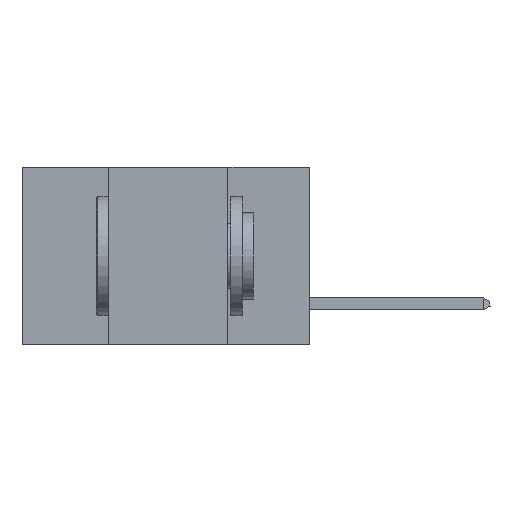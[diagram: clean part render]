
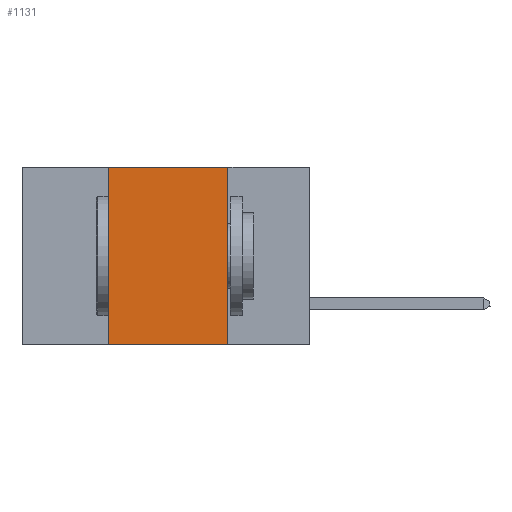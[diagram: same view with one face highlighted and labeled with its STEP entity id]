
A CAD part, left-side view. The second image highlights one B-rep face of the part: STEP entity #1131.
In plain terms, the highlighted planar face has unit normal (-1, 0, 0).
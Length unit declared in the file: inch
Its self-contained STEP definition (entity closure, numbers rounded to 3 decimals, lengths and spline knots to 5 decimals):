
#219 = VERTEX_POINT ( 'NONE', #9685 ) ;
#1131 = ADVANCED_FACE ( 'NONE', ( #25147 ), #12726, .F. ) ;
#2560 = CARTESIAN_POINT ( 'NONE',  ( 0., 0.42, 0. ) ) ;
#2862 = DIRECTION ( 'NONE',  ( 0., -1., 0. ) ) ;
#3616 = ORIENTED_EDGE ( 'NONE', *, *, #7091, .T. ) ;
#6191 = LINE ( 'NONE', #12866, #13840 ) ;
#6233 = DIRECTION ( 'NONE',  ( 0., 0., -1. ) ) ;
#6569 = DIRECTION ( 'NONE',  ( 0., 0., 1. ) ) ;
#7091 = EDGE_CURVE ( 'NONE', #219, #16683, #10833, .T. ) ;
#7781 = VERTEX_POINT ( 'NONE', #19347 ) ;
#8742 = CARTESIAN_POINT ( 'NONE',  ( 0., 0.6, 0. ) ) ;
#9492 = AXIS2_PLACEMENT_3D ( 'NONE', #16805, #12630, #6233 ) ;
#9685 = CARTESIAN_POINT ( 'NONE',  ( 0., 0.42, -0.37 ) ) ;
#10094 = VECTOR ( 'NONE', #6569, 39.37008 ) ;
#10508 = VECTOR ( 'NONE', #24185, 39.37008 ) ;
#10833 = LINE ( 'NONE', #14062, #10508 ) ;
#12136 = EDGE_CURVE ( 'NONE', #219, #7781, #21481, .T. ) ;
#12630 = DIRECTION ( 'NONE',  ( 1., 0., 0. ) ) ;
#12726 = PLANE ( 'NONE',  #9492 ) ;
#12866 = CARTESIAN_POINT ( 'NONE',  ( 0., 0.17, 0. ) ) ;
#13433 = VECTOR ( 'NONE', #2862, 39.37008 ) ;
#13840 = VECTOR ( 'NONE', #14814, 39.37008 ) ;
#14062 = CARTESIAN_POINT ( 'NONE',  ( 0., 0.6, -0.37 ) ) ;
#14814 = DIRECTION ( 'NONE',  ( 0., 0., -1. ) ) ;
#15110 = EDGE_CURVE ( 'NONE', #7781, #15606, #25733, .T. ) ;
#15606 = VERTEX_POINT ( 'NONE', #24855 ) ;
#16683 = VERTEX_POINT ( 'NONE', #23047 ) ;
#16805 = CARTESIAN_POINT ( 'NONE',  ( 0., 0.6, 0. ) ) ;
#17158 = EDGE_LOOP ( 'NONE', ( #20463, #25442, #21222, #3616 ) ) ;
#19347 = CARTESIAN_POINT ( 'NONE',  ( 0., 0.42, 0. ) ) ;
#20463 = ORIENTED_EDGE ( 'NONE', *, *, #26202, .F. ) ;
#21222 = ORIENTED_EDGE ( 'NONE', *, *, #12136, .F. ) ;
#21481 = LINE ( 'NONE', #2560, #10094 ) ;
#23047 = CARTESIAN_POINT ( 'NONE',  ( 0., 0.17, -0.37 ) ) ;
#24185 = DIRECTION ( 'NONE',  ( 0., -1., 0. ) ) ;
#24855 = CARTESIAN_POINT ( 'NONE',  ( 0., 0.17, 0. ) ) ;
#25147 = FACE_OUTER_BOUND ( 'NONE', #17158, .T. ) ;
#25442 = ORIENTED_EDGE ( 'NONE', *, *, #15110, .F. ) ;
#25733 = LINE ( 'NONE', #8742, #13433 ) ;
#26202 = EDGE_CURVE ( 'NONE', #15606, #16683, #6191, .T. ) ;
